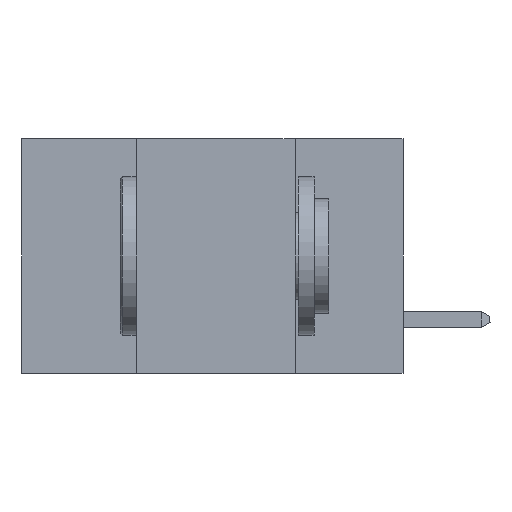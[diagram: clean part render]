
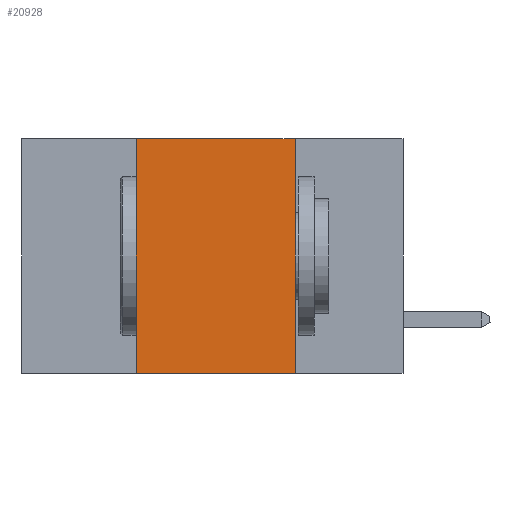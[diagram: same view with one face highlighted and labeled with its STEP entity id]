
A CAD part, left-side view. The second image highlights one B-rep face of the part: STEP entity #20928.
In plain terms, the highlighted planar face has unit normal (-1, 0, 0).
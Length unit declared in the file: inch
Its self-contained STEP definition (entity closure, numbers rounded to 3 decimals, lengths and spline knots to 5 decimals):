
#90 = ORIENTED_EDGE ( 'NONE', *, *, #726, .F. ) ;
#405 = AXIS2_PLACEMENT_3D ( 'NONE', #9674, #20788, #15070 ) ;
#433 = PLANE ( 'NONE',  #405 ) ;
#686 = LINE ( 'NONE', #5776, #4757 ) ;
#726 = EDGE_CURVE ( 'NONE', #9228, #2901, #17830, .T. ) ;
#1122 = CARTESIAN_POINT ( 'NONE',  ( 0., 0.42, 0. ) ) ;
#1782 = VECTOR ( 'NONE', #20225, 39.37008 ) ;
#2606 = CARTESIAN_POINT ( 'NONE',  ( 0., 0.42, -0.37 ) ) ;
#2901 = VERTEX_POINT ( 'NONE', #1122 ) ;
#3004 = EDGE_CURVE ( 'NONE', #9083, #21368, #10471, .T. ) ;
#4757 = VECTOR ( 'NONE', #13148, 39.37008 ) ;
#5156 = FACE_OUTER_BOUND ( 'NONE', #22087, .T. ) ;
#5776 = CARTESIAN_POINT ( 'NONE',  ( 0., 0.6, -0.37 ) ) ;
#6576 = ORIENTED_EDGE ( 'NONE', *, *, #9073, .T. ) ;
#6705 = CARTESIAN_POINT ( 'NONE',  ( 0., 0.17, -0.37 ) ) ;
#7037 = ORIENTED_EDGE ( 'NONE', *, *, #3004, .F. ) ;
#7486 = CARTESIAN_POINT ( 'NONE',  ( 0., 0.17, 0. ) ) ;
#9073 = EDGE_CURVE ( 'NONE', #9228, #21368, #686, .T. ) ;
#9083 = VERTEX_POINT ( 'NONE', #7486 ) ;
#9228 = VERTEX_POINT ( 'NONE', #2606 ) ;
#9674 = CARTESIAN_POINT ( 'NONE',  ( 0., 0.6, 0. ) ) ;
#10471 = LINE ( 'NONE', #21806, #15343 ) ;
#12112 = VECTOR ( 'NONE', #21323, 39.37008 ) ;
#12190 = CARTESIAN_POINT ( 'NONE',  ( 0., 0.6, 0. ) ) ;
#12812 = CARTESIAN_POINT ( 'NONE',  ( 0., 0.42, 0. ) ) ;
#13148 = DIRECTION ( 'NONE',  ( 0., -1., 0. ) ) ;
#13267 = LINE ( 'NONE', #12190, #12112 ) ;
#13699 = EDGE_CURVE ( 'NONE', #2901, #9083, #13267, .T. ) ;
#15070 = DIRECTION ( 'NONE',  ( 0., 0., -1. ) ) ;
#15343 = VECTOR ( 'NONE', #16356, 39.37008 ) ;
#16356 = DIRECTION ( 'NONE',  ( 0., 0., -1. ) ) ;
#17830 = LINE ( 'NONE', #12812, #1782 ) ;
#20225 = DIRECTION ( 'NONE',  ( 0., 0., 1. ) ) ;
#20788 = DIRECTION ( 'NONE',  ( 1., 0., 0. ) ) ;
#20928 = ADVANCED_FACE ( 'NONE', ( #5156 ), #433, .F. ) ;
#21323 = DIRECTION ( 'NONE',  ( 0., -1., 0. ) ) ;
#21368 = VERTEX_POINT ( 'NONE', #6705 ) ;
#21806 = CARTESIAN_POINT ( 'NONE',  ( 0., 0.17, 0. ) ) ;
#22087 = EDGE_LOOP ( 'NONE', ( #7037, #23606, #90, #6576 ) ) ;
#23606 = ORIENTED_EDGE ( 'NONE', *, *, #13699, .F. ) ;
